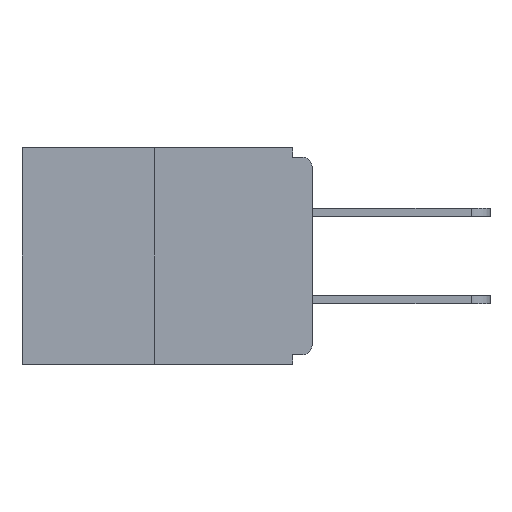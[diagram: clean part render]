
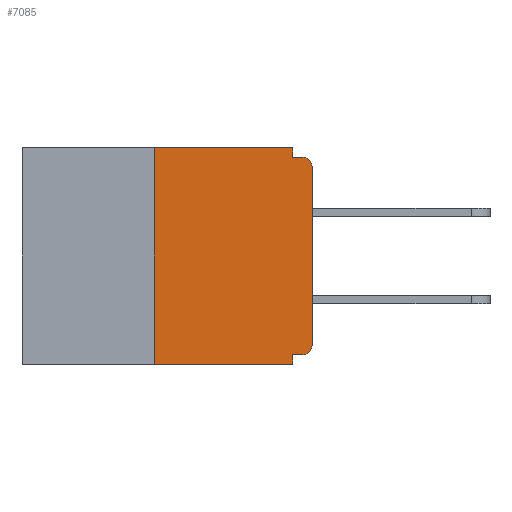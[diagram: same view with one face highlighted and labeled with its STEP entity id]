
A CAD part, left-side view. The second image highlights one B-rep face of the part: STEP entity #7085.
In plain terms, the highlighted planar face has unit normal (-1, 0, 0).
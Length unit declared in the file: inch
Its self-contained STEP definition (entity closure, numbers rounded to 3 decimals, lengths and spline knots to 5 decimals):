
#343 = CARTESIAN_POINT ( 'NONE',  ( 0., 0., 0. ) ) ;
#620 = LINE ( 'NONE', #17604, #19401 ) ;
#956 = DIRECTION ( 'NONE',  ( -1., 0., 0. ) ) ;
#1082 = DIRECTION ( 'NONE',  ( 0., 0., 1. ) ) ;
#1448 = CARTESIAN_POINT ( 'NONE',  ( 0., 0.015, -0.03 ) ) ;
#1528 = DIRECTION ( 'NONE',  ( 0., 0., -1. ) ) ;
#2620 = VECTOR ( 'NONE', #18587, 39.37008 ) ;
#2677 = CARTESIAN_POINT ( 'NONE',  ( 0., 0.25, 0. ) ) ;
#2909 = LINE ( 'NONE', #343, #2620 ) ;
#3631 = LINE ( 'NONE', #11718, #4184 ) ;
#4184 = VECTOR ( 'NONE', #4517, 39.37008 ) ;
#4341 = CIRCLE ( 'NONE', #5085, 0.015 ) ;
#4514 = CARTESIAN_POINT ( 'NONE',  ( 0., 0.015, -0.313 ) ) ;
#4517 = DIRECTION ( 'NONE',  ( 0., 1., 0. ) ) ;
#4563 = DIRECTION ( 'NONE',  ( 0., -1., 0. ) ) ;
#5085 = AXIS2_PLACEMENT_3D ( 'NONE', #1448, #15909, #1528 ) ;
#5120 = VERTEX_POINT ( 'NONE', #17498 ) ;
#5578 = VECTOR ( 'NONE', #1082, 39.37008 ) ;
#6170 = EDGE_CURVE ( 'NONE', #9755, #8955, #17365, .T. ) ;
#6210 = DIRECTION ( 'NONE',  ( 0., -1., 0. ) ) ;
#6275 = ORIENTED_EDGE ( 'NONE', *, *, #18575, .F. ) ;
#6454 = EDGE_CURVE ( 'NONE', #8955, #5120, #21061, .T. ) ;
#7085 = ADVANCED_FACE ( 'NONE', ( #20154 ), #15765, .F. ) ;
#7500 = ORIENTED_EDGE ( 'NONE', *, *, #12129, .F. ) ;
#7671 = VECTOR ( 'NONE', #4563, 39.37008 ) ;
#7829 = EDGE_CURVE ( 'NONE', #9148, #9324, #2909, .T. ) ;
#8397 = CARTESIAN_POINT ( 'NONE',  ( 0., 0.031, -0.343 ) ) ;
#8502 = DIRECTION ( 'NONE',  ( 0., 0., -1. ) ) ;
#8641 = ORIENTED_EDGE ( 'NONE', *, *, #20590, .T. ) ;
#8955 = VERTEX_POINT ( 'NONE', #22680 ) ;
#8965 = VERTEX_POINT ( 'NONE', #13562 ) ;
#8985 = CARTESIAN_POINT ( 'NONE',  ( 0., 0.25, 0. ) ) ;
#9067 = VECTOR ( 'NONE', #6210, 39.37008 ) ;
#9148 = VERTEX_POINT ( 'NONE', #21636 ) ;
#9195 = EDGE_LOOP ( 'NONE', ( #18022, #7500, #19044, #6275, #14876, #8641, #9717, #9427, #10684, #20554 ) ) ;
#9324 = VERTEX_POINT ( 'NONE', #22411 ) ;
#9427 = ORIENTED_EDGE ( 'NONE', *, *, #13895, .T. ) ;
#9717 = ORIENTED_EDGE ( 'NONE', *, *, #7829, .T. ) ;
#9755 = VERTEX_POINT ( 'NONE', #8985 ) ;
#10499 = VERTEX_POINT ( 'NONE', #14979 ) ;
#10684 = ORIENTED_EDGE ( 'NONE', *, *, #15261, .F. ) ;
#11206 = CARTESIAN_POINT ( 'NONE',  ( 0., 0., -0.015 ) ) ;
#11688 = CARTESIAN_POINT ( 'NONE',  ( 0., 0.46, 0. ) ) ;
#11718 = CARTESIAN_POINT ( 'NONE',  ( 0., 0., -0.328 ) ) ;
#11772 = LINE ( 'NONE', #2677, #5578 ) ;
#12129 = EDGE_CURVE ( 'NONE', #22006, #9755, #11772, .T. ) ;
#12140 = DIRECTION ( 'NONE',  ( 0., 0., -1. ) ) ;
#12287 = AXIS2_PLACEMENT_3D ( 'NONE', #13977, #17697, #8502 ) ;
#12801 = AXIS2_PLACEMENT_3D ( 'NONE', #4514, #956, #13614 ) ;
#13562 = CARTESIAN_POINT ( 'NONE',  ( 0., 0.031, -0.328 ) ) ;
#13614 = DIRECTION ( 'NONE',  ( 0., 0., -1. ) ) ;
#13895 = EDGE_CURVE ( 'NONE', #9324, #23444, #4341, .T. ) ;
#13977 = CARTESIAN_POINT ( 'NONE',  ( 0., 0.46, 0. ) ) ;
#14517 = DIRECTION ( 'NONE',  ( 0., -1., 0. ) ) ;
#14769 = LINE ( 'NONE', #11206, #9067 ) ;
#14876 = ORIENTED_EDGE ( 'NONE', *, *, #23464, .F. ) ;
#14979 = CARTESIAN_POINT ( 'NONE',  ( 0., 0.015, -0.328 ) ) ;
#15261 = EDGE_CURVE ( 'NONE', #5120, #23444, #14769, .T. ) ;
#15488 = CIRCLE ( 'NONE', #12801, 0.015 ) ;
#15765 = PLANE ( 'NONE',  #12287 ) ;
#15909 = DIRECTION ( 'NONE',  ( -1., 0., 0. ) ) ;
#15935 = EDGE_CURVE ( 'NONE', #22006, #21361, #16191, .T. ) ;
#16191 = LINE ( 'NONE', #16316, #17332 ) ;
#16316 = CARTESIAN_POINT ( 'NONE',  ( 0., 0.46, -0.343 ) ) ;
#17332 = VECTOR ( 'NONE', #14517, 39.37008 ) ;
#17365 = LINE ( 'NONE', #11688, #7671 ) ;
#17498 = CARTESIAN_POINT ( 'NONE',  ( 0., 0.031, -0.015 ) ) ;
#17604 = CARTESIAN_POINT ( 'NONE',  ( 0., 0.031, -0.343 ) ) ;
#17697 = DIRECTION ( 'NONE',  ( 1., 0., 0. ) ) ;
#18022 = ORIENTED_EDGE ( 'NONE', *, *, #6170, .F. ) ;
#18575 = EDGE_CURVE ( 'NONE', #8965, #21361, #620, .T. ) ;
#18587 = DIRECTION ( 'NONE',  ( 0., 0., 1. ) ) ;
#18788 = VECTOR ( 'NONE', #23357, 39.37008 ) ;
#18929 = CARTESIAN_POINT ( 'NONE',  ( 0., 0.015, -0.015 ) ) ;
#19044 = ORIENTED_EDGE ( 'NONE', *, *, #15935, .T. ) ;
#19130 = CARTESIAN_POINT ( 'NONE',  ( 0., 0.031, 0. ) ) ;
#19401 = VECTOR ( 'NONE', #12140, 39.37008 ) ;
#20154 = FACE_OUTER_BOUND ( 'NONE', #9195, .T. ) ;
#20554 = ORIENTED_EDGE ( 'NONE', *, *, #6454, .F. ) ;
#20590 = EDGE_CURVE ( 'NONE', #10499, #9148, #15488, .T. ) ;
#21061 = LINE ( 'NONE', #19130, #18788 ) ;
#21361 = VERTEX_POINT ( 'NONE', #8397 ) ;
#21636 = CARTESIAN_POINT ( 'NONE',  ( 0., 0., -0.313 ) ) ;
#22006 = VERTEX_POINT ( 'NONE', #22323 ) ;
#22323 = CARTESIAN_POINT ( 'NONE',  ( 0., 0.25, -0.343 ) ) ;
#22411 = CARTESIAN_POINT ( 'NONE',  ( 0., 0., -0.03 ) ) ;
#22680 = CARTESIAN_POINT ( 'NONE',  ( 0., 0.031, 0. ) ) ;
#23357 = DIRECTION ( 'NONE',  ( 0., 0., -1. ) ) ;
#23444 = VERTEX_POINT ( 'NONE', #18929 ) ;
#23464 = EDGE_CURVE ( 'NONE', #10499, #8965, #3631, .T. ) ;
